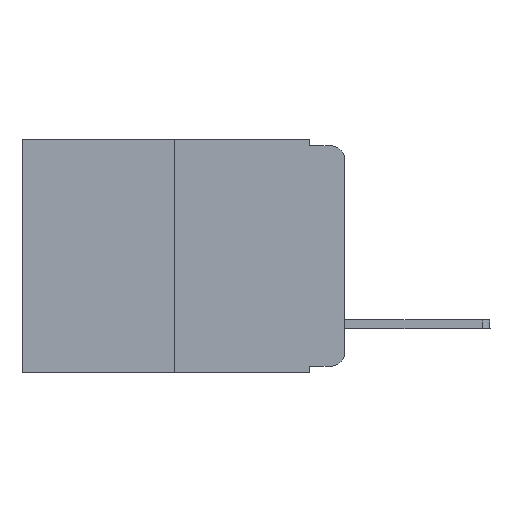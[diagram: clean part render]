
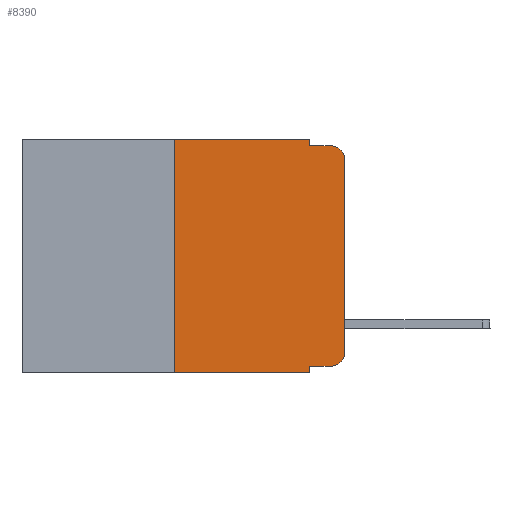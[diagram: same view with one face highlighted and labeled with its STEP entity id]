
A CAD part, left-side view. The second image highlights one B-rep face of the part: STEP entity #8390.
In plain terms, the highlighted planar face has unit normal (-1, 0, 0).
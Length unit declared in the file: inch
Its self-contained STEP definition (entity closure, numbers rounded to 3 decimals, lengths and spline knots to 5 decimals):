
#310 = CARTESIAN_POINT ( 'NONE',  ( 0., 0.051, 0. ) ) ;
#491 = DIRECTION ( 'NONE',  ( 0., 0., -1. ) ) ;
#886 = LINE ( 'NONE', #2698, #7264 ) ;
#904 = CARTESIAN_POINT ( 'NONE',  ( 0., 0.02, -0.01 ) ) ;
#1010 = DIRECTION ( 'NONE',  ( 0., -1., 0. ) ) ;
#1066 = CARTESIAN_POINT ( 'NONE',  ( 0., 0.051, 0. ) ) ;
#1131 = EDGE_CURVE ( 'NONE', #7572, #5447, #6466, .T. ) ;
#1363 = EDGE_CURVE ( 'NONE', #2108, #3073, #9325, .T. ) ;
#1531 = ORIENTED_EDGE ( 'NONE', *, *, #8706, .F. ) ;
#1580 = CARTESIAN_POINT ( 'NONE',  ( 0., 0.051, -0.01 ) ) ;
#1753 = VECTOR ( 'NONE', #4207, 39.37008 ) ;
#2108 = VERTEX_POINT ( 'NONE', #310 ) ;
#2167 = ORIENTED_EDGE ( 'NONE', *, *, #1131, .T. ) ;
#2490 = CARTESIAN_POINT ( 'NONE',  ( 0., 0.051, 0. ) ) ;
#2563 = DIRECTION ( 'NONE',  ( 0., 0., -1. ) ) ;
#2606 = VERTEX_POINT ( 'NONE', #904 ) ;
#2631 = CARTESIAN_POINT ( 'NONE',  ( 0., 0.473, -0.343 ) ) ;
#2656 = LINE ( 'NONE', #9177, #1753 ) ;
#2698 = CARTESIAN_POINT ( 'NONE',  ( 0., 0.25, 0. ) ) ;
#2740 = PLANE ( 'NONE',  #3676 ) ;
#2849 = CARTESIAN_POINT ( 'NONE',  ( 0., 0.02, -0.313 ) ) ;
#3032 = FACE_OUTER_BOUND ( 'NONE', #7265, .T. ) ;
#3060 = CIRCLE ( 'NONE', #3446, 0.02 ) ;
#3073 = VERTEX_POINT ( 'NONE', #1580 ) ;
#3236 = VERTEX_POINT ( 'NONE', #7901 ) ;
#3415 = ORIENTED_EDGE ( 'NONE', *, *, #6605, .T. ) ;
#3443 = VECTOR ( 'NONE', #1010, 39.37008 ) ;
#3446 = AXIS2_PLACEMENT_3D ( 'NONE', #6912, #3633, #10287 ) ;
#3449 = DIRECTION ( 'NONE',  ( 0., 0., 1. ) ) ;
#3545 = ORIENTED_EDGE ( 'NONE', *, *, #8341, .F. ) ;
#3612 = CARTESIAN_POINT ( 'NONE',  ( 0., 0.051, -0.343 ) ) ;
#3633 = DIRECTION ( 'NONE',  ( -1., 0., 0. ) ) ;
#3676 = AXIS2_PLACEMENT_3D ( 'NONE', #6103, #6009, #6838 ) ;
#4207 = DIRECTION ( 'NONE',  ( 0., -1., 0. ) ) ;
#4262 = VECTOR ( 'NONE', #5558, 39.37008 ) ;
#4352 = LINE ( 'NONE', #2490, #6826 ) ;
#4427 = ORIENTED_EDGE ( 'NONE', *, *, #1363, .F. ) ;
#4438 = AXIS2_PLACEMENT_3D ( 'NONE', #2849, #6178, #491 ) ;
#4986 = VERTEX_POINT ( 'NONE', #7477 ) ;
#5288 = VERTEX_POINT ( 'NONE', #7581 ) ;
#5447 = VERTEX_POINT ( 'NONE', #8483 ) ;
#5558 = DIRECTION ( 'NONE',  ( 0., -1., 0. ) ) ;
#5587 = VERTEX_POINT ( 'NONE', #3612 ) ;
#5647 = LINE ( 'NONE', #10142, #3443 ) ;
#5886 = ORIENTED_EDGE ( 'NONE', *, *, #9260, .T. ) ;
#6009 = DIRECTION ( 'NONE',  ( 1., 0., 0. ) ) ;
#6055 = CIRCLE ( 'NONE', #4438, 0.02 ) ;
#6103 = CARTESIAN_POINT ( 'NONE',  ( 0., 0.473, 0. ) ) ;
#6178 = DIRECTION ( 'NONE',  ( -1., 0., 0. ) ) ;
#6311 = ORIENTED_EDGE ( 'NONE', *, *, #6625, .F. ) ;
#6466 = LINE ( 'NONE', #8105, #4262 ) ;
#6605 = EDGE_CURVE ( 'NONE', #3236, #2606, #3060, .T. ) ;
#6625 = EDGE_CURVE ( 'NONE', #5288, #7952, #886, .T. ) ;
#6727 = CARTESIAN_POINT ( 'NONE',  ( 0., 0., 0. ) ) ;
#6826 = VECTOR ( 'NONE', #2563, 39.37008 ) ;
#6838 = DIRECTION ( 'NONE',  ( 0., 0., -1. ) ) ;
#6878 = DIRECTION ( 'NONE',  ( 0., 0., -1. ) ) ;
#6910 = ORIENTED_EDGE ( 'NONE', *, *, #8357, .T. ) ;
#6912 = CARTESIAN_POINT ( 'NONE',  ( 0., 0.02, -0.03 ) ) ;
#7125 = ORIENTED_EDGE ( 'NONE', *, *, #8876, .T. ) ;
#7218 = CARTESIAN_POINT ( 'NONE',  ( 0., 0.051, -0.333 ) ) ;
#7264 = VECTOR ( 'NONE', #8569, 39.37008 ) ;
#7265 = EDGE_LOOP ( 'NONE', ( #6910, #3415, #1531, #4427, #3545, #6311, #5886, #10375, #2167, #7125 ) ) ;
#7477 = CARTESIAN_POINT ( 'NONE',  ( 0., 0., -0.313 ) ) ;
#7572 = VERTEX_POINT ( 'NONE', #7218 ) ;
#7581 = CARTESIAN_POINT ( 'NONE',  ( 0., 0.25, -0.343 ) ) ;
#7901 = CARTESIAN_POINT ( 'NONE',  ( 0., 0., -0.03 ) ) ;
#7952 = VERTEX_POINT ( 'NONE', #9444 ) ;
#8105 = CARTESIAN_POINT ( 'NONE',  ( 0., 0.051, -0.333 ) ) ;
#8341 = EDGE_CURVE ( 'NONE', #7952, #2108, #2656, .T. ) ;
#8357 = EDGE_CURVE ( 'NONE', #4986, #3236, #8780, .T. ) ;
#8390 = ADVANCED_FACE ( 'NONE', ( #3032 ), #2740, .F. ) ;
#8483 = CARTESIAN_POINT ( 'NONE',  ( 0., 0.02, -0.333 ) ) ;
#8569 = DIRECTION ( 'NONE',  ( 0., 0., 1. ) ) ;
#8706 = EDGE_CURVE ( 'NONE', #3073, #2606, #5647, .T. ) ;
#8780 = LINE ( 'NONE', #6727, #10723 ) ;
#8876 = EDGE_CURVE ( 'NONE', #5447, #4986, #6055, .T. ) ;
#8880 = LINE ( 'NONE', #2631, #10567 ) ;
#9118 = EDGE_CURVE ( 'NONE', #7572, #5587, #4352, .T. ) ;
#9177 = CARTESIAN_POINT ( 'NONE',  ( 0., 0.473, 0. ) ) ;
#9260 = EDGE_CURVE ( 'NONE', #5288, #5587, #8880, .T. ) ;
#9325 = LINE ( 'NONE', #1066, #9698 ) ;
#9412 = DIRECTION ( 'NONE',  ( 0., -1., 0. ) ) ;
#9444 = CARTESIAN_POINT ( 'NONE',  ( 0., 0.25, 0. ) ) ;
#9698 = VECTOR ( 'NONE', #6878, 39.37008 ) ;
#10142 = CARTESIAN_POINT ( 'NONE',  ( 0., 0.051, -0.01 ) ) ;
#10287 = DIRECTION ( 'NONE',  ( 0., 0., -1. ) ) ;
#10375 = ORIENTED_EDGE ( 'NONE', *, *, #9118, .F. ) ;
#10567 = VECTOR ( 'NONE', #9412, 39.37008 ) ;
#10723 = VECTOR ( 'NONE', #3449, 39.37008 ) ;
